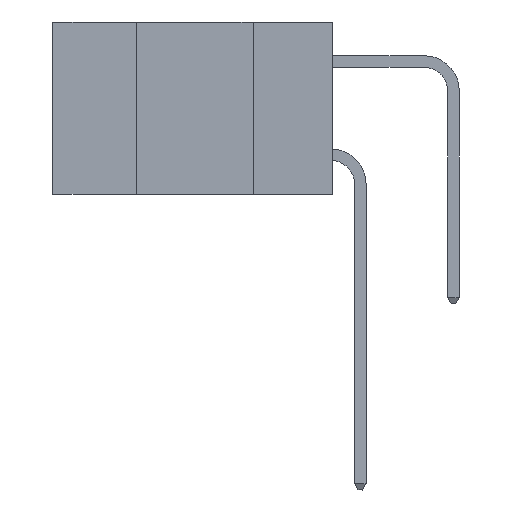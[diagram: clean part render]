
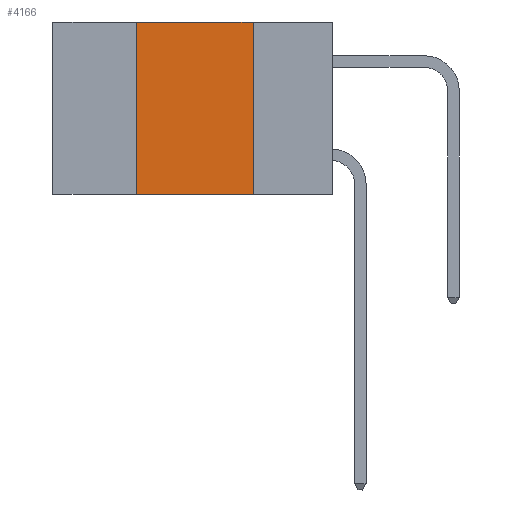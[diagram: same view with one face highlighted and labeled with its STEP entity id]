
A CAD part, left-side view. The second image highlights one B-rep face of the part: STEP entity #4166.
In plain terms, the highlighted planar face has unit normal (-1, 0, 0).
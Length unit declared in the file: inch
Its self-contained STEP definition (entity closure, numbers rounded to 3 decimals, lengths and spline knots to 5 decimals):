
#20 = DIRECTION ( 'NONE',  ( 0., -1., 0. ) ) ;
#347 = ORIENTED_EDGE ( 'NONE', *, *, #1048, .T. ) ;
#684 = CARTESIAN_POINT ( 'NONE',  ( 0., 0.17, 0. ) ) ;
#857 = PLANE ( 'NONE',  #12696 ) ;
#968 = LINE ( 'NONE', #13416, #8784 ) ;
#973 = CARTESIAN_POINT ( 'NONE',  ( 0., 0.17, -0.37 ) ) ;
#1048 = EDGE_CURVE ( 'NONE', #9809, #9236, #2045, .T. ) ;
#1681 = DIRECTION ( 'NONE',  ( 0., 0., -1. ) ) ;
#1847 = VERTEX_POINT ( 'NONE', #5636 ) ;
#2045 = LINE ( 'NONE', #3436, #7630 ) ;
#3038 = ORIENTED_EDGE ( 'NONE', *, *, #10178, .F. ) ;
#3436 = CARTESIAN_POINT ( 'NONE',  ( 0., 0.6, -0.37 ) ) ;
#3689 = FACE_OUTER_BOUND ( 'NONE', #7928, .T. ) ;
#4166 = ADVANCED_FACE ( 'NONE', ( #3689 ), #857, .F. ) ;
#4173 = ORIENTED_EDGE ( 'NONE', *, *, #11545, .F. ) ;
#4615 = LINE ( 'NONE', #4999, #12421 ) ;
#4999 = CARTESIAN_POINT ( 'NONE',  ( 0., 0.42, 0. ) ) ;
#5399 = CARTESIAN_POINT ( 'NONE',  ( 0., 0.6, 0. ) ) ;
#5636 = CARTESIAN_POINT ( 'NONE',  ( 0., 0.42, 0. ) ) ;
#5742 = DIRECTION ( 'NONE',  ( 0., -1., 0. ) ) ;
#5853 = CARTESIAN_POINT ( 'NONE',  ( 0., 0.42, -0.37 ) ) ;
#6116 = LINE ( 'NONE', #684, #12182 ) ;
#7221 = CARTESIAN_POINT ( 'NONE',  ( 0., 0.17, 0. ) ) ;
#7630 = VECTOR ( 'NONE', #20, 39.37008 ) ;
#7676 = DIRECTION ( 'NONE',  ( 0., 0., -1. ) ) ;
#7739 = VERTEX_POINT ( 'NONE', #7221 ) ;
#7928 = EDGE_LOOP ( 'NONE', ( #14070, #3038, #4173, #347 ) ) ;
#8784 = VECTOR ( 'NONE', #5742, 39.37008 ) ;
#9236 = VERTEX_POINT ( 'NONE', #973 ) ;
#9809 = VERTEX_POINT ( 'NONE', #5853 ) ;
#10178 = EDGE_CURVE ( 'NONE', #1847, #7739, #968, .T. ) ;
#10450 = DIRECTION ( 'NONE',  ( 0., 0., 1. ) ) ;
#11545 = EDGE_CURVE ( 'NONE', #9809, #1847, #4615, .T. ) ;
#12182 = VECTOR ( 'NONE', #1681, 39.37008 ) ;
#12421 = VECTOR ( 'NONE', #10450, 39.37008 ) ;
#12696 = AXIS2_PLACEMENT_3D ( 'NONE', #5399, #14268, #7676 ) ;
#13416 = CARTESIAN_POINT ( 'NONE',  ( 0., 0.6, 0. ) ) ;
#14070 = ORIENTED_EDGE ( 'NONE', *, *, #14123, .F. ) ;
#14123 = EDGE_CURVE ( 'NONE', #7739, #9236, #6116, .T. ) ;
#14268 = DIRECTION ( 'NONE',  ( 1., 0., 0. ) ) ;
